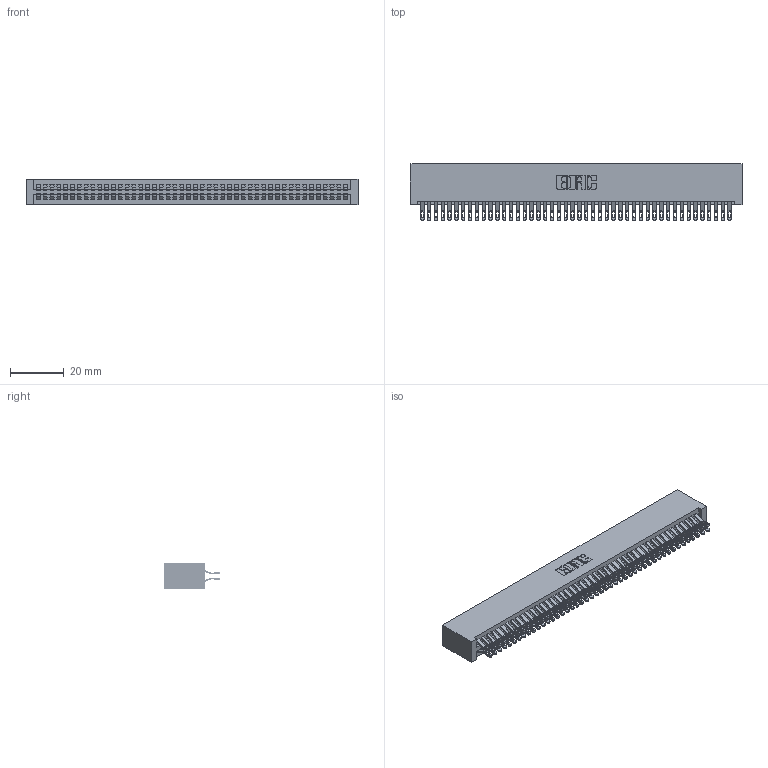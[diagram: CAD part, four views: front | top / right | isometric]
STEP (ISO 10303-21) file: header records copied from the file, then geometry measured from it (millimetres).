
FILE_DESCRIPTION (( 'STEP AP203' ), '1' );
FILE_NAME ('395-092-555-201.STEP', '2018-11-29T08:38:26', ( '' ), ( '' ), 'SwSTEP 2.0', 'SolidWorks 2016', '' );
FILE_SCHEMA (( 'CONFIG_CONTROL_DESIGN' ));
Length unit declared in the file: inch
Products named in the file (3): 395-092-555-201; 345 Part_No Mounting Lugs; 345-292-001_555 Tail
Assembly tree (93 placements, depth 2):
  395-092-555-201
    345 Part_No Mounting Lugs
    345-292-001_555 Tail  x92
Bounding box: 123.44 x 21.13 x 9.4 mm (x, y, z)
Volume: 12911.4 mm3; surface area: 20394 mm2
Topology: 93 solids, 93 shells, 5270 faces, 16601 edges, 11066 vertices
Faces by surface type: plane 2928, cylinder 2342
Entity records: 35603 total; most frequent: CARTESIAN_POINT 5998, ORIENTED_EDGE 5902, DIRECTION 5247, EDGE_CURVE 2951, VECTOR 2623, LINE 2623, VERTEX_POINT 1966, AXIS2_PLACEMENT_3D 1312
